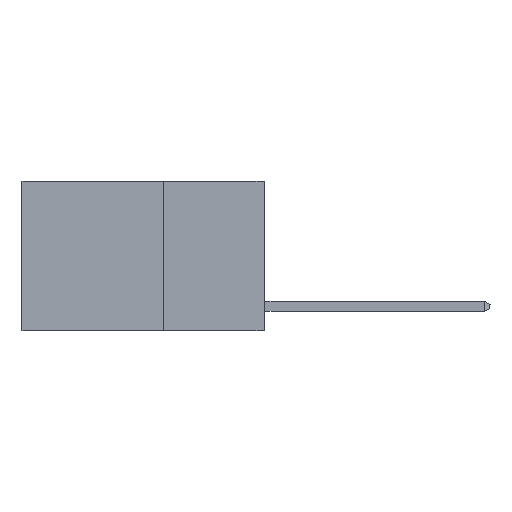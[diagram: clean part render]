
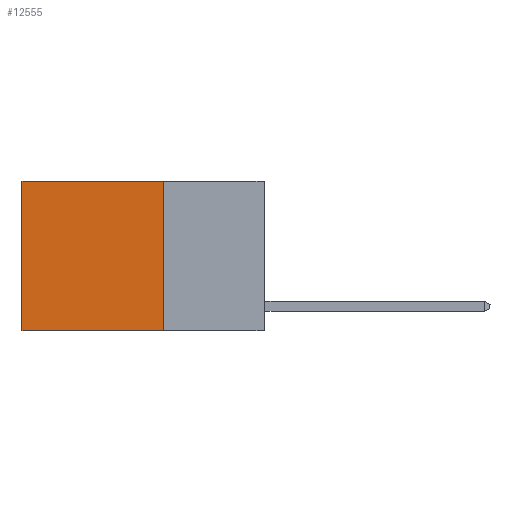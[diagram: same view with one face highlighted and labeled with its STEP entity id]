
A CAD part, left-side view. The second image highlights one B-rep face of the part: STEP entity #12555.
In plain terms, the highlighted planar face has unit normal (-1, 0, 0).
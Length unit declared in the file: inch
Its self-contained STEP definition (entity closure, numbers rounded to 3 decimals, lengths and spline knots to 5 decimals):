
#424 = EDGE_CURVE ( 'NONE', #16371, #21062, #17059, .T. ) ;
#764 = EDGE_CURVE ( 'NONE', #5178, #16371, #20389, .T. ) ;
#923 = EDGE_CURVE ( 'NONE', #5178, #2165, #6551, .T. ) ;
#1572 = CARTESIAN_POINT ( 'NONE',  ( 0.2625, 0.25, -0.37 ) ) ;
#2165 = VERTEX_POINT ( 'NONE', #1572 ) ;
#3217 = DIRECTION ( 'NONE',  ( 0., 0., -1. ) ) ;
#3903 = ORIENTED_EDGE ( 'NONE', *, *, #764, .T. ) ;
#4269 = EDGE_LOOP ( 'NONE', ( #20059, #19024, #12958, #3903 ) ) ;
#4790 = VECTOR ( 'NONE', #13382, 39.37008 ) ;
#5150 = DIRECTION ( 'NONE',  ( 0., 0., -1. ) ) ;
#5178 = VERTEX_POINT ( 'NONE', #17405 ) ;
#6551 = LINE ( 'NONE', #12470, #17735 ) ;
#7680 = CARTESIAN_POINT ( 'NONE',  ( 0.2625, 0.6, 0. ) ) ;
#8713 = CARTESIAN_POINT ( 'NONE',  ( 0.2625, 0.6, -0.37 ) ) ;
#8911 = DIRECTION ( 'NONE',  ( 1., 0., 0. ) ) ;
#10432 = CARTESIAN_POINT ( 'NONE',  ( 0.2625, 0.25, -0.37 ) ) ;
#10496 = AXIS2_PLACEMENT_3D ( 'NONE', #14512, #8911, #5150 ) ;
#12066 = DIRECTION ( 'NONE',  ( 0., 1., 0. ) ) ;
#12470 = CARTESIAN_POINT ( 'NONE',  ( 0.2625, 0.25, 0. ) ) ;
#12555 = ADVANCED_FACE ( 'NONE', ( #22154 ), #20072, .F. ) ;
#12958 = ORIENTED_EDGE ( 'NONE', *, *, #923, .F. ) ;
#13382 = DIRECTION ( 'NONE',  ( 0., 0., -1. ) ) ;
#14512 = CARTESIAN_POINT ( 'NONE',  ( 0.2625, 0.25, 0. ) ) ;
#14646 = VECTOR ( 'NONE', #22343, 39.37008 ) ;
#14826 = CARTESIAN_POINT ( 'NONE',  ( 0.2625, 0.25, 0. ) ) ;
#16371 = VERTEX_POINT ( 'NONE', #7680 ) ;
#17059 = LINE ( 'NONE', #20546, #4790 ) ;
#17405 = CARTESIAN_POINT ( 'NONE',  ( 0.2625, 0.25, 0. ) ) ;
#17734 = EDGE_CURVE ( 'NONE', #2165, #21062, #23552, .T. ) ;
#17735 = VECTOR ( 'NONE', #3217, 39.37008 ) ;
#19024 = ORIENTED_EDGE ( 'NONE', *, *, #17734, .F. ) ;
#20059 = ORIENTED_EDGE ( 'NONE', *, *, #424, .T. ) ;
#20072 = PLANE ( 'NONE',  #10496 ) ;
#20389 = LINE ( 'NONE', #14826, #14646 ) ;
#20457 = VECTOR ( 'NONE', #12066, 39.37008 ) ;
#20546 = CARTESIAN_POINT ( 'NONE',  ( 0.2625, 0.6, 0. ) ) ;
#21062 = VERTEX_POINT ( 'NONE', #8713 ) ;
#22154 = FACE_OUTER_BOUND ( 'NONE', #4269, .T. ) ;
#22343 = DIRECTION ( 'NONE',  ( 0., 1., 0. ) ) ;
#23552 = LINE ( 'NONE', #10432, #20457 ) ;
